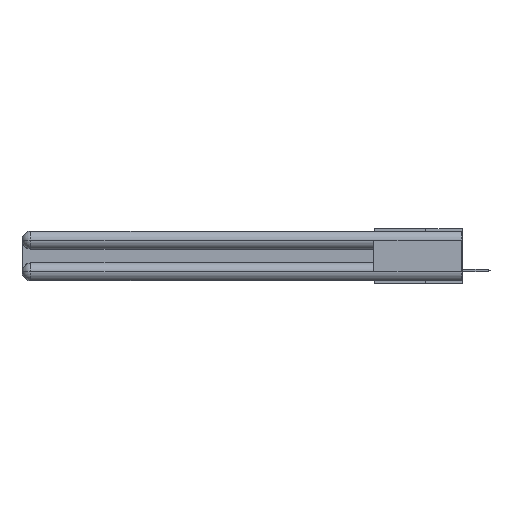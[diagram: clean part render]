
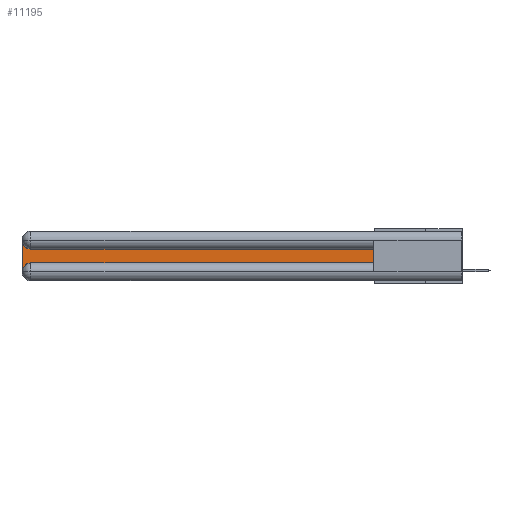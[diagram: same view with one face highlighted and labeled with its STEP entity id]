
A CAD part, left-side view. The second image highlights one B-rep face of the part: STEP entity #11195.
In plain terms, the highlighted planar face has unit normal (-1, 0, 0).
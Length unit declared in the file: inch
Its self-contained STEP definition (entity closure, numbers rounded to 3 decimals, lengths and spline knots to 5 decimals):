
#1172 = DIRECTION ( 'NONE',  ( 0., 1., 0. ) ) ;
#1981 = CARTESIAN_POINT ( 'NONE',  ( 0.075, 2.94, -0.2175 ) ) ;
#3263 = DIRECTION ( 'NONE',  ( 1., 0., 0. ) ) ;
#4364 = VECTOR ( 'NONE', #16593, 39.37008 ) ;
#4534 = AXIS2_PLACEMENT_3D ( 'NONE', #15675, #23865, #31559 ) ;
#4761 = LINE ( 'NONE', #22589, #26486 ) ;
#5224 = VERTEX_POINT ( 'NONE', #26939 ) ;
#6330 = EDGE_CURVE ( 'NONE', #28275, #5224, #11618, .T. ) ;
#7741 = VERTEX_POINT ( 'NONE', #8847 ) ;
#8606 = VECTOR ( 'NONE', #21937, 39.37008 ) ;
#8642 = CARTESIAN_POINT ( 'NONE',  ( 0.075, 3., -0.2775 ) ) ;
#8847 = CARTESIAN_POINT ( 'NONE',  ( 0.075, 0.6, -0.1225 ) ) ;
#9011 = EDGE_CURVE ( 'NONE', #5224, #19664, #10700, .T. ) ;
#9775 = CARTESIAN_POINT ( 'NONE',  ( 0.075, 2.94, -0.0625 ) ) ;
#10168 = PLANE ( 'NONE',  #4534 ) ;
#10700 = LINE ( 'NONE', #32838, #8606 ) ;
#10710 = AXIS2_PLACEMENT_3D ( 'NONE', #9775, #23376, #17864 ) ;
#10757 = VERTEX_POINT ( 'NONE', #1981 ) ;
#11195 = ADVANCED_FACE ( 'NONE', ( #27811 ), #10168, .F. ) ;
#11618 = CIRCLE ( 'NONE', #10710, 0.06 ) ;
#13044 = ORIENTED_EDGE ( 'NONE', *, *, #19206, .T. ) ;
#14018 = CARTESIAN_POINT ( 'NONE',  ( 0.075, 2.94, -0.2775 ) ) ;
#14111 = CIRCLE ( 'NONE', #20150, 0.06 ) ;
#14761 = ORIENTED_EDGE ( 'NONE', *, *, #6330, .T. ) ;
#15675 = CARTESIAN_POINT ( 'NONE',  ( 0.075, 3., -0.1225 ) ) ;
#16290 = ORIENTED_EDGE ( 'NONE', *, *, #9011, .T. ) ;
#16593 = DIRECTION ( 'NONE',  ( 0., 0., 1. ) ) ;
#17315 = LINE ( 'NONE', #21888, #4364 ) ;
#17864 = DIRECTION ( 'NONE',  ( 0., 0., -1. ) ) ;
#18364 = EDGE_CURVE ( 'NONE', #19664, #10757, #14111, .T. ) ;
#18469 = DIRECTION ( 'NONE',  ( 0., -1., 0. ) ) ;
#18853 = CARTESIAN_POINT ( 'NONE',  ( 0.075, 2.94, -0.1225 ) ) ;
#19206 = EDGE_CURVE ( 'NONE', #10757, #30952, #33714, .T. ) ;
#19664 = VERTEX_POINT ( 'NONE', #8642 ) ;
#20150 = AXIS2_PLACEMENT_3D ( 'NONE', #14018, #3263, #29994 ) ;
#20681 = ORIENTED_EDGE ( 'NONE', *, *, #28788, .T. ) ;
#21888 = CARTESIAN_POINT ( 'NONE',  ( 0.075, 0.6, -0.2175 ) ) ;
#21937 = DIRECTION ( 'NONE',  ( 0., 0., -1. ) ) ;
#22589 = CARTESIAN_POINT ( 'NONE',  ( 0.075, 0.6, -0.1225 ) ) ;
#23376 = DIRECTION ( 'NONE',  ( 1., 0., 0. ) ) ;
#23528 = ORIENTED_EDGE ( 'NONE', *, *, #29407, .T. ) ;
#23865 = DIRECTION ( 'NONE',  ( 1., 0., 0. ) ) ;
#25889 = ORIENTED_EDGE ( 'NONE', *, *, #18364, .T. ) ;
#26486 = VECTOR ( 'NONE', #1172, 39.37008 ) ;
#26593 = CARTESIAN_POINT ( 'NONE',  ( 0.075, 0.6, -0.2175 ) ) ;
#26700 = CARTESIAN_POINT ( 'NONE',  ( 0.075, 0.6, -0.2175 ) ) ;
#26939 = CARTESIAN_POINT ( 'NONE',  ( 0.075, 3., -0.0625 ) ) ;
#27811 = FACE_OUTER_BOUND ( 'NONE', #31710, .T. ) ;
#28275 = VERTEX_POINT ( 'NONE', #18853 ) ;
#28788 = EDGE_CURVE ( 'NONE', #7741, #28275, #4761, .T. ) ;
#29407 = EDGE_CURVE ( 'NONE', #30952, #7741, #17315, .T. ) ;
#29994 = DIRECTION ( 'NONE',  ( 0., 0., -1. ) ) ;
#30952 = VERTEX_POINT ( 'NONE', #26593 ) ;
#31207 = VECTOR ( 'NONE', #18469, 39.37008 ) ;
#31559 = DIRECTION ( 'NONE',  ( 0., 0., -1. ) ) ;
#31710 = EDGE_LOOP ( 'NONE', ( #20681, #14761, #16290, #25889, #13044, #23528 ) ) ;
#32838 = CARTESIAN_POINT ( 'NONE',  ( 0.075, 3., -0.2175 ) ) ;
#33714 = LINE ( 'NONE', #26700, #31207 ) ;
